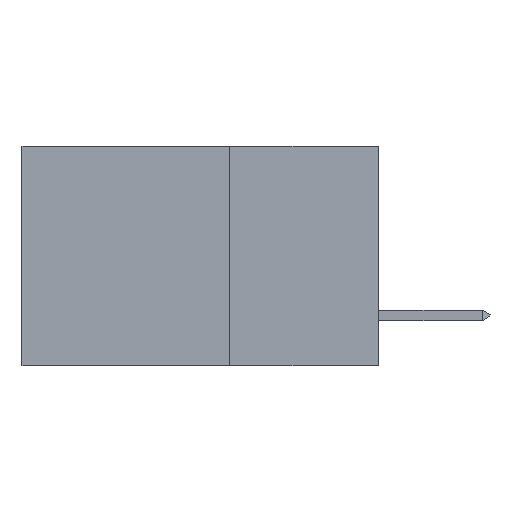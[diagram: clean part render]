
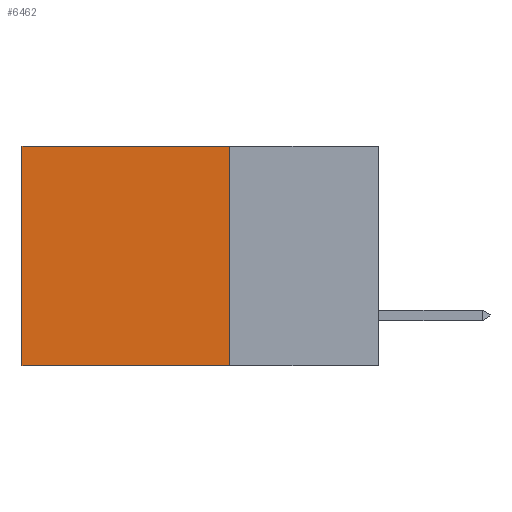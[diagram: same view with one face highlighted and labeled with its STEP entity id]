
A CAD part, left-side view. The second image highlights one B-rep face of the part: STEP entity #6462.
In plain terms, the highlighted planar face has unit normal (-1, 0, 0).
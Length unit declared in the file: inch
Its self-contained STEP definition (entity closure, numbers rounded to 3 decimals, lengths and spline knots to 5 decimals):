
#91 = CARTESIAN_POINT ( 'NONE',  ( 0.298, 0.25, -0.37 ) ) ;
#400 = EDGE_LOOP ( 'NONE', ( #8634, #7052, #8599, #5372 ) ) ;
#998 = VERTEX_POINT ( 'NONE', #10962 ) ;
#1578 = CARTESIAN_POINT ( 'NONE',  ( 0.298, 0.6, 0. ) ) ;
#1613 = LINE ( 'NONE', #9005, #3949 ) ;
#2123 = PLANE ( 'NONE',  #2726 ) ;
#2610 = EDGE_CURVE ( 'NONE', #6534, #6871, #4552, .T. ) ;
#2726 = AXIS2_PLACEMENT_3D ( 'NONE', #5551, #5653, #5593 ) ;
#3834 = VECTOR ( 'NONE', #9523, 39.37008 ) ;
#3949 = VECTOR ( 'NONE', #7231, 39.37008 ) ;
#4552 = LINE ( 'NONE', #1578, #5068 ) ;
#5068 = VECTOR ( 'NONE', #10153, 39.37008 ) ;
#5120 = CARTESIAN_POINT ( 'NONE',  ( 0.298, 0.6, -0.37 ) ) ;
#5372 = ORIENTED_EDGE ( 'NONE', *, *, #9131, .T. ) ;
#5551 = CARTESIAN_POINT ( 'NONE',  ( 0.298, 0.25, 0. ) ) ;
#5593 = DIRECTION ( 'NONE',  ( 0., 0., -1. ) ) ;
#5653 = DIRECTION ( 'NONE',  ( 1., 0., 0. ) ) ;
#6090 = LINE ( 'NONE', #6654, #3834 ) ;
#6462 = ADVANCED_FACE ( 'NONE', ( #9041 ), #2123, .F. ) ;
#6534 = VERTEX_POINT ( 'NONE', #6679 ) ;
#6557 = DIRECTION ( 'NONE',  ( 0., 0., -1. ) ) ;
#6654 = CARTESIAN_POINT ( 'NONE',  ( 0.298, 0.25, 0. ) ) ;
#6679 = CARTESIAN_POINT ( 'NONE',  ( 0.298, 0.6, 0. ) ) ;
#6684 = EDGE_CURVE ( 'NONE', #998, #8744, #9598, .T. ) ;
#6871 = VERTEX_POINT ( 'NONE', #5120 ) ;
#7052 = ORIENTED_EDGE ( 'NONE', *, *, #8914, .F. ) ;
#7118 = CARTESIAN_POINT ( 'NONE',  ( 0.298, 0.25, 0. ) ) ;
#7231 = DIRECTION ( 'NONE',  ( 0., 1., 0. ) ) ;
#8599 = ORIENTED_EDGE ( 'NONE', *, *, #6684, .F. ) ;
#8634 = ORIENTED_EDGE ( 'NONE', *, *, #2610, .T. ) ;
#8744 = VERTEX_POINT ( 'NONE', #91 ) ;
#8914 = EDGE_CURVE ( 'NONE', #8744, #6871, #1613, .T. ) ;
#9005 = CARTESIAN_POINT ( 'NONE',  ( 0.298, 0.25, -0.37 ) ) ;
#9041 = FACE_OUTER_BOUND ( 'NONE', #400, .T. ) ;
#9131 = EDGE_CURVE ( 'NONE', #998, #6534, #6090, .T. ) ;
#9523 = DIRECTION ( 'NONE',  ( 0., 1., 0. ) ) ;
#9598 = LINE ( 'NONE', #7118, #10690 ) ;
#10153 = DIRECTION ( 'NONE',  ( 0., 0., -1. ) ) ;
#10690 = VECTOR ( 'NONE', #6557, 39.37008 ) ;
#10962 = CARTESIAN_POINT ( 'NONE',  ( 0.298, 0.25, 0. ) ) ;
